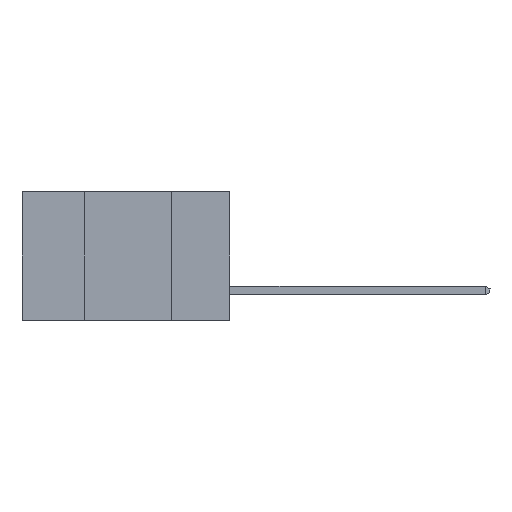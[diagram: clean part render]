
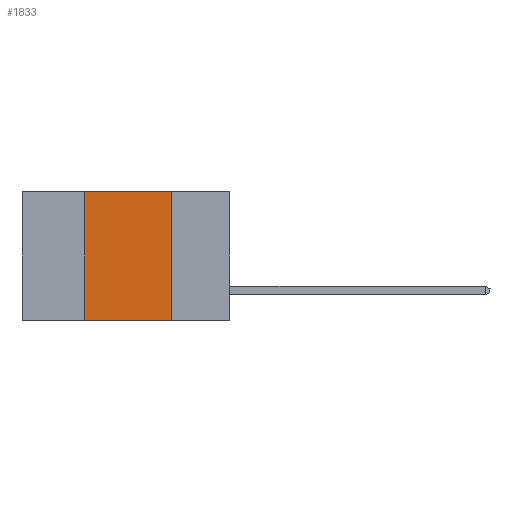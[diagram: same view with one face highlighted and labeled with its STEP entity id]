
A CAD part, left-side view. The second image highlights one B-rep face of the part: STEP entity #1833.
In plain terms, the highlighted planar face has unit normal (-1, 0, 0).
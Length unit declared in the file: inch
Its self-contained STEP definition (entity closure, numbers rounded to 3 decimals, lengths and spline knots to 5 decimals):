
#1833 = ADVANCED_FACE ( 'NONE', ( #4834 ), #14838, .F. ) ;
#2199 = DIRECTION ( 'NONE',  ( 0., 0., 1. ) ) ;
#2235 = DIRECTION ( 'NONE',  ( 0., 0., -1. ) ) ;
#3482 = DIRECTION ( 'NONE',  ( 0., 0., -1. ) ) ;
#4188 = VECTOR ( 'NONE', #12661, 39.37008 ) ;
#4207 = CARTESIAN_POINT ( 'NONE',  ( 0., 0.6, 0. ) ) ;
#4834 = FACE_OUTER_BOUND ( 'NONE', #7745, .T. ) ;
#5424 = VERTEX_POINT ( 'NONE', #15343 ) ;
#5692 = ORIENTED_EDGE ( 'NONE', *, *, #15991, .F. ) ;
#6345 = VECTOR ( 'NONE', #2199, 39.37008 ) ;
#7198 = ORIENTED_EDGE ( 'NONE', *, *, #10203, .F. ) ;
#7517 = LINE ( 'NONE', #12597, #12349 ) ;
#7745 = EDGE_LOOP ( 'NONE', ( #7198, #11456, #5692, #14270 ) ) ;
#8763 = LINE ( 'NONE', #13826, #4188 ) ;
#8821 = CARTESIAN_POINT ( 'NONE',  ( 0., 0.42, -0.37 ) ) ;
#9504 = VERTEX_POINT ( 'NONE', #10774 ) ;
#9842 = DIRECTION ( 'NONE',  ( 1., 0., 0. ) ) ;
#10203 = EDGE_CURVE ( 'NONE', #14983, #11149, #7517, .T. ) ;
#10774 = CARTESIAN_POINT ( 'NONE',  ( 0., 0.42, 0. ) ) ;
#11110 = VECTOR ( 'NONE', #16181, 39.37008 ) ;
#11149 = VERTEX_POINT ( 'NONE', #12619 ) ;
#11183 = LINE ( 'NONE', #4207, #11110 ) ;
#11456 = ORIENTED_EDGE ( 'NONE', *, *, #16353, .F. ) ;
#12349 = VECTOR ( 'NONE', #2235, 39.37008 ) ;
#12597 = CARTESIAN_POINT ( 'NONE',  ( 0., 0.17, -0.37 ) ) ;
#12619 = CARTESIAN_POINT ( 'NONE',  ( 0., 0.17, -0.37 ) ) ;
#12638 = AXIS2_PLACEMENT_3D ( 'NONE', #13747, #9842, #3482 ) ;
#12661 = DIRECTION ( 'NONE',  ( 0., -1., 0. ) ) ;
#13630 = LINE ( 'NONE', #8821, #6345 ) ;
#13747 = CARTESIAN_POINT ( 'NONE',  ( 0., 0.6, 0. ) ) ;
#13826 = CARTESIAN_POINT ( 'NONE',  ( 0., 0.6, -0.37 ) ) ;
#14270 = ORIENTED_EDGE ( 'NONE', *, *, #15586, .T. ) ;
#14838 = PLANE ( 'NONE',  #12638 ) ;
#14983 = VERTEX_POINT ( 'NONE', #15688 ) ;
#15343 = CARTESIAN_POINT ( 'NONE',  ( 0., 0.42, -0.37 ) ) ;
#15586 = EDGE_CURVE ( 'NONE', #5424, #11149, #8763, .T. ) ;
#15688 = CARTESIAN_POINT ( 'NONE',  ( 0., 0.17, 0. ) ) ;
#15991 = EDGE_CURVE ( 'NONE', #5424, #9504, #13630, .T. ) ;
#16181 = DIRECTION ( 'NONE',  ( 0., -1., 0. ) ) ;
#16353 = EDGE_CURVE ( 'NONE', #9504, #14983, #11183, .T. ) ;
